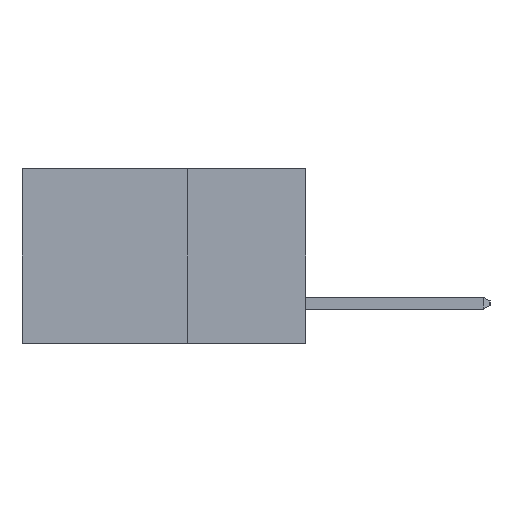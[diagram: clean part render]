
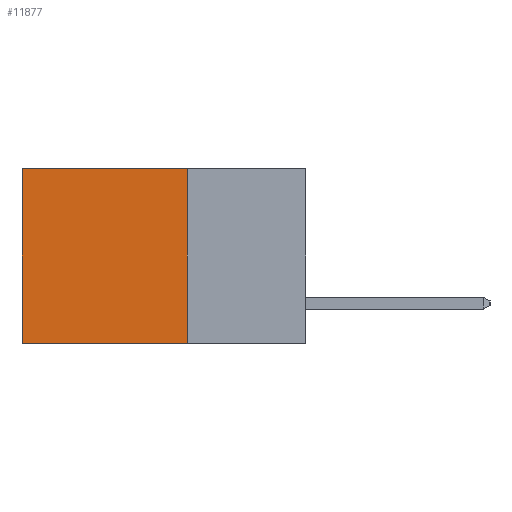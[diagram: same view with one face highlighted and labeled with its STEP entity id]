
A CAD part, left-side view. The second image highlights one B-rep face of the part: STEP entity #11877.
In plain terms, the highlighted planar face has unit normal (-1, 0, 0).
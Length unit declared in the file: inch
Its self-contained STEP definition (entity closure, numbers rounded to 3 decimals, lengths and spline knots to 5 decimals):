
#751 = LINE ( 'NONE', #4810, #14272 ) ;
#2452 = ORIENTED_EDGE ( 'NONE', *, *, #9712, .F. ) ;
#2515 = VECTOR ( 'NONE', #5635, 39.37008 ) ;
#3307 = PLANE ( 'NONE',  #6519 ) ;
#3595 = EDGE_CURVE ( 'NONE', #10261, #10605, #11204, .T. ) ;
#3992 = ORIENTED_EDGE ( 'NONE', *, *, #4564, .F. ) ;
#4315 = ORIENTED_EDGE ( 'NONE', *, *, #5567, .T. ) ;
#4564 = EDGE_CURVE ( 'NONE', #4982, #9998, #751, .T. ) ;
#4810 = CARTESIAN_POINT ( 'NONE',  ( 0.298, 0.25, -0.37 ) ) ;
#4912 = DIRECTION ( 'NONE',  ( 1., 0., 0. ) ) ;
#4982 = VERTEX_POINT ( 'NONE', #12305 ) ;
#5567 = EDGE_CURVE ( 'NONE', #10605, #9998, #7003, .T. ) ;
#5635 = DIRECTION ( 'NONE',  ( 0., 0., -1. ) ) ;
#6100 = VECTOR ( 'NONE', #18195, 39.37008 ) ;
#6519 = AXIS2_PLACEMENT_3D ( 'NONE', #12641, #4912, #15767 ) ;
#7003 = LINE ( 'NONE', #19581, #18753 ) ;
#8663 = FACE_OUTER_BOUND ( 'NONE', #13503, .T. ) ;
#9712 = EDGE_CURVE ( 'NONE', #10261, #4982, #15946, .T. ) ;
#9998 = VERTEX_POINT ( 'NONE', #18620 ) ;
#10261 = VERTEX_POINT ( 'NONE', #14685 ) ;
#10605 = VERTEX_POINT ( 'NONE', #13279 ) ;
#11133 = DIRECTION ( 'NONE',  ( 0., 1., 0. ) ) ;
#11204 = LINE ( 'NONE', #14109, #6100 ) ;
#11877 = ADVANCED_FACE ( 'NONE', ( #8663 ), #3307, .F. ) ;
#12305 = CARTESIAN_POINT ( 'NONE',  ( 0.298, 0.25, -0.37 ) ) ;
#12641 = CARTESIAN_POINT ( 'NONE',  ( 0.298, 0.25, 0. ) ) ;
#13279 = CARTESIAN_POINT ( 'NONE',  ( 0.298, 0.6, 0. ) ) ;
#13503 = EDGE_LOOP ( 'NONE', ( #4315, #3992, #2452, #14584 ) ) ;
#14109 = CARTESIAN_POINT ( 'NONE',  ( 0.298, 0.25, 0. ) ) ;
#14272 = VECTOR ( 'NONE', #11133, 39.37008 ) ;
#14584 = ORIENTED_EDGE ( 'NONE', *, *, #3595, .T. ) ;
#14685 = CARTESIAN_POINT ( 'NONE',  ( 0.298, 0.25, 0. ) ) ;
#15767 = DIRECTION ( 'NONE',  ( 0., 0., -1. ) ) ;
#15946 = LINE ( 'NONE', #16476, #2515 ) ;
#16476 = CARTESIAN_POINT ( 'NONE',  ( 0.298, 0.25, 0. ) ) ;
#18195 = DIRECTION ( 'NONE',  ( 0., 1., 0. ) ) ;
#18620 = CARTESIAN_POINT ( 'NONE',  ( 0.298, 0.6, -0.37 ) ) ;
#18753 = VECTOR ( 'NONE', #19015, 39.37008 ) ;
#19015 = DIRECTION ( 'NONE',  ( 0., 0., -1. ) ) ;
#19581 = CARTESIAN_POINT ( 'NONE',  ( 0.298, 0.6, 0. ) ) ;
